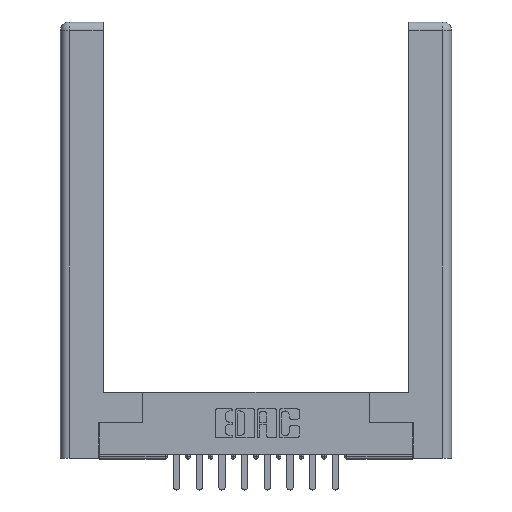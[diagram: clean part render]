
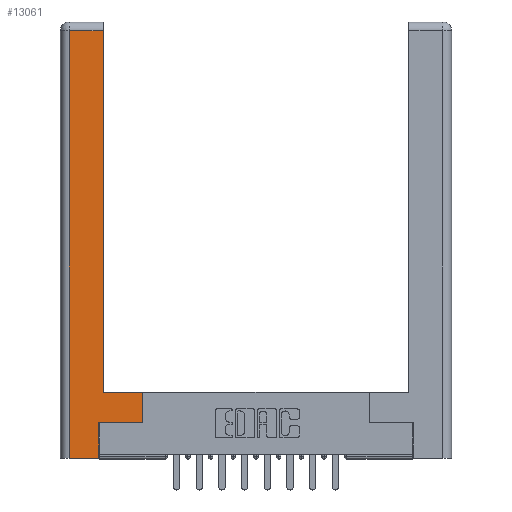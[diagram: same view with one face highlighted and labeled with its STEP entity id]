
A CAD part, top view. The second image highlights one B-rep face of the part: STEP entity #13061.
In plain terms, the highlighted planar face has unit normal (0, 0, 1).
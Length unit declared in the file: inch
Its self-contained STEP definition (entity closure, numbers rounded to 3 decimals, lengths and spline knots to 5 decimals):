
#78 = VERTEX_POINT ( 'NONE', #10518 ) ;
#91 = CARTESIAN_POINT ( 'NONE',  ( 0.265, 0.245, 0. ) ) ;
#511 = EDGE_CURVE ( 'NONE', #1634, #6462, #4579, .T. ) ;
#523 = CARTESIAN_POINT ( 'NONE',  ( 0.295, 0.45, 0. ) ) ;
#835 = CARTESIAN_POINT ( 'NONE',  ( 0.265, 0.245, 0. ) ) ;
#836 = DIRECTION ( 'NONE',  ( 0., -1., 0. ) ) ;
#1084 = VERTEX_POINT ( 'NONE', #6364 ) ;
#1094 = LINE ( 'NONE', #6795, #4443 ) ;
#1107 = EDGE_CURVE ( 'NONE', #78, #1634, #9734, .T. ) ;
#1634 = VERTEX_POINT ( 'NONE', #12393 ) ;
#1930 = ORIENTED_EDGE ( 'NONE', *, *, #9789, .T. ) ;
#1965 = LINE ( 'NONE', #5471, #14181 ) ;
#2155 = EDGE_CURVE ( 'NONE', #5930, #1084, #6725, .T. ) ;
#2205 = PLANE ( 'NONE',  #2981 ) ;
#2309 = CARTESIAN_POINT ( 'NONE',  ( 0.565, 0.245, 0. ) ) ;
#2481 = CARTESIAN_POINT ( 'NONE',  ( 0.565, 0.245, 0. ) ) ;
#2981 = AXIS2_PLACEMENT_3D ( 'NONE', #13828, #6967, #6756 ) ;
#2994 = LINE ( 'NONE', #7188, #12439 ) ;
#3763 = FACE_OUTER_BOUND ( 'NONE', #12832, .T. ) ;
#3829 = VECTOR ( 'NONE', #14929, 39.37008 ) ;
#4188 = ORIENTED_EDGE ( 'NONE', *, *, #10986, .T. ) ;
#4443 = VECTOR ( 'NONE', #836, 39.37008 ) ;
#4579 = LINE ( 'NONE', #5061, #3829 ) ;
#5061 = CARTESIAN_POINT ( 'NONE',  ( 0.295, 3., 0. ) ) ;
#5471 = CARTESIAN_POINT ( 'NONE',  ( 0.0615, 2.94, 0. ) ) ;
#5930 = VERTEX_POINT ( 'NONE', #9667 ) ;
#6364 = CARTESIAN_POINT ( 'NONE',  ( 0.265, 0., 0. ) ) ;
#6462 = VERTEX_POINT ( 'NONE', #8288 ) ;
#6725 = LINE ( 'NONE', #7883, #10822 ) ;
#6756 = DIRECTION ( 'NONE',  ( -1., 0., 0. ) ) ;
#6795 = CARTESIAN_POINT ( 'NONE',  ( 0.0615, 0., 0. ) ) ;
#6918 = EDGE_CURVE ( 'NONE', #6462, #10683, #1965, .T. ) ;
#6967 = DIRECTION ( 'NONE',  ( 0., 0., -1. ) ) ;
#7130 = DIRECTION ( 'NONE',  ( 0., 1., 0. ) ) ;
#7188 = CARTESIAN_POINT ( 'NONE',  ( 0.565, 0.45, 0. ) ) ;
#7670 = VERTEX_POINT ( 'NONE', #91 ) ;
#7883 = CARTESIAN_POINT ( 'NONE',  ( 0.265, 0., 0. ) ) ;
#8288 = CARTESIAN_POINT ( 'NONE',  ( 0.295, 2.94, 0. ) ) ;
#8503 = LINE ( 'NONE', #835, #11322 ) ;
#9158 = EDGE_CURVE ( 'NONE', #7670, #12105, #14277, .T. ) ;
#9271 = ORIENTED_EDGE ( 'NONE', *, *, #511, .T. ) ;
#9667 = CARTESIAN_POINT ( 'NONE',  ( 0.0615, 0., 0. ) ) ;
#9725 = DIRECTION ( 'NONE',  ( 1., 0., 0. ) ) ;
#9734 = LINE ( 'NONE', #523, #14524 ) ;
#9789 = EDGE_CURVE ( 'NONE', #12105, #78, #2994, .T. ) ;
#9838 = ORIENTED_EDGE ( 'NONE', *, *, #2155, .T. ) ;
#10311 = DIRECTION ( 'NONE',  ( 0., 1., 0. ) ) ;
#10518 = CARTESIAN_POINT ( 'NONE',  ( 0.565, 0.45, 0. ) ) ;
#10683 = VERTEX_POINT ( 'NONE', #12582 ) ;
#10822 = VECTOR ( 'NONE', #13953, 39.37008 ) ;
#10986 = EDGE_CURVE ( 'NONE', #10683, #5930, #1094, .T. ) ;
#11322 = VECTOR ( 'NONE', #10311, 39.37008 ) ;
#11413 = ORIENTED_EDGE ( 'NONE', *, *, #6918, .T. ) ;
#12062 = ORIENTED_EDGE ( 'NONE', *, *, #1107, .T. ) ;
#12105 = VERTEX_POINT ( 'NONE', #2481 ) ;
#12393 = CARTESIAN_POINT ( 'NONE',  ( 0.295, 0.45, 0. ) ) ;
#12439 = VECTOR ( 'NONE', #7130, 39.37008 ) ;
#12582 = CARTESIAN_POINT ( 'NONE',  ( 0.0615, 2.94, 0. ) ) ;
#12711 = DIRECTION ( 'NONE',  ( -1., 0., 0. ) ) ;
#12832 = EDGE_LOOP ( 'NONE', ( #9271, #11413, #4188, #9838, #13484, #14328, #1930, #12062 ) ) ;
#13061 = ADVANCED_FACE ( 'NONE', ( #3763 ), #2205, .F. ) ;
#13219 = EDGE_CURVE ( 'NONE', #1084, #7670, #8503, .T. ) ;
#13484 = ORIENTED_EDGE ( 'NONE', *, *, #13219, .T. ) ;
#13828 = CARTESIAN_POINT ( 'NONE',  ( 0., 0., 0. ) ) ;
#13953 = DIRECTION ( 'NONE',  ( 1., 0., 0. ) ) ;
#14181 = VECTOR ( 'NONE', #12711, 39.37008 ) ;
#14277 = LINE ( 'NONE', #2309, #15028 ) ;
#14328 = ORIENTED_EDGE ( 'NONE', *, *, #9158, .T. ) ;
#14524 = VECTOR ( 'NONE', #14747, 39.37008 ) ;
#14747 = DIRECTION ( 'NONE',  ( -1., 0., 0. ) ) ;
#14929 = DIRECTION ( 'NONE',  ( 0., 1., 0. ) ) ;
#15028 = VECTOR ( 'NONE', #9725, 39.37008 ) ;
